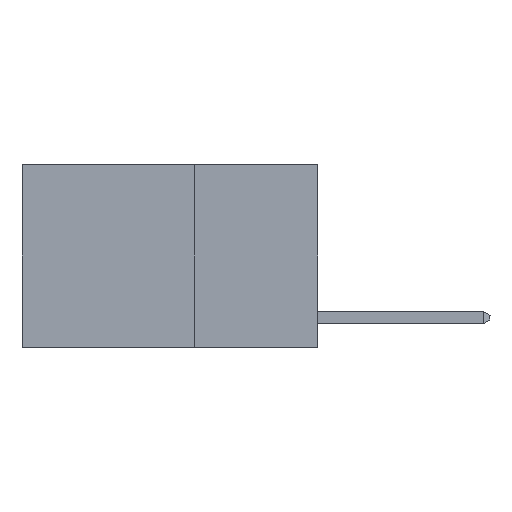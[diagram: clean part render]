
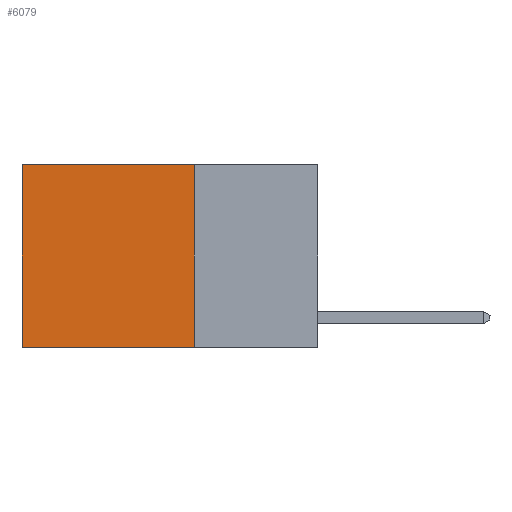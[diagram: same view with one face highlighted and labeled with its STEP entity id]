
A CAD part, left-side view. The second image highlights one B-rep face of the part: STEP entity #6079.
In plain terms, the highlighted planar face has unit normal (-1, 0, 0).
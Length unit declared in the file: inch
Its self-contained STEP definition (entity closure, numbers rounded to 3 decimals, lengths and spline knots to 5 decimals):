
#65 = LINE ( 'NONE', #15000, #6848 ) ;
#456 = VERTEX_POINT ( 'NONE', #9681 ) ;
#506 = EDGE_CURVE ( 'NONE', #2422, #10743, #3334, .T. ) ;
#2422 = VERTEX_POINT ( 'NONE', #9698 ) ;
#2647 = EDGE_CURVE ( 'NONE', #456, #5254, #65, .T. ) ;
#2948 = VECTOR ( 'NONE', #9373, 39.37008 ) ;
#2974 = ORIENTED_EDGE ( 'NONE', *, *, #14936, .F. ) ;
#2992 = DIRECTION ( 'NONE',  ( 0., 0., -1. ) ) ;
#3334 = LINE ( 'NONE', #9472, #2948 ) ;
#3987 = DIRECTION ( 'NONE',  ( 1., 0., 0. ) ) ;
#4174 = LINE ( 'NONE', #11429, #4573 ) ;
#4189 = ORIENTED_EDGE ( 'NONE', *, *, #7579, .T. ) ;
#4573 = VECTOR ( 'NONE', #2992, 39.37008 ) ;
#5254 = VERTEX_POINT ( 'NONE', #10690 ) ;
#6079 = ADVANCED_FACE ( 'NONE', ( #9887 ), #11171, .F. ) ;
#6286 = AXIS2_PLACEMENT_3D ( 'NONE', #8864, #3987, #12351 ) ;
#6848 = VECTOR ( 'NONE', #14938, 39.37008 ) ;
#7579 = EDGE_CURVE ( 'NONE', #5254, #10743, #13871, .T. ) ;
#7671 = VECTOR ( 'NONE', #13179, 39.37008 ) ;
#8773 = ORIENTED_EDGE ( 'NONE', *, *, #506, .F. ) ;
#8809 = ORIENTED_EDGE ( 'NONE', *, *, #2647, .T. ) ;
#8864 = CARTESIAN_POINT ( 'NONE',  ( 0.2625, 0.25, 0. ) ) ;
#9373 = DIRECTION ( 'NONE',  ( 0., 1., 0. ) ) ;
#9472 = CARTESIAN_POINT ( 'NONE',  ( 0.2625, 0.25, -0.37 ) ) ;
#9681 = CARTESIAN_POINT ( 'NONE',  ( 0.2625, 0.25, 0. ) ) ;
#9698 = CARTESIAN_POINT ( 'NONE',  ( 0.2625, 0.25, -0.37 ) ) ;
#9887 = FACE_OUTER_BOUND ( 'NONE', #11472, .T. ) ;
#10690 = CARTESIAN_POINT ( 'NONE',  ( 0.2625, 0.6, 0. ) ) ;
#10743 = VERTEX_POINT ( 'NONE', #13209 ) ;
#11171 = PLANE ( 'NONE',  #6286 ) ;
#11429 = CARTESIAN_POINT ( 'NONE',  ( 0.2625, 0.25, 0. ) ) ;
#11472 = EDGE_LOOP ( 'NONE', ( #4189, #8773, #2974, #8809 ) ) ;
#11949 = CARTESIAN_POINT ( 'NONE',  ( 0.2625, 0.6, 0. ) ) ;
#12351 = DIRECTION ( 'NONE',  ( 0., 0., -1. ) ) ;
#13179 = DIRECTION ( 'NONE',  ( 0., 0., -1. ) ) ;
#13209 = CARTESIAN_POINT ( 'NONE',  ( 0.2625, 0.6, -0.37 ) ) ;
#13871 = LINE ( 'NONE', #11949, #7671 ) ;
#14936 = EDGE_CURVE ( 'NONE', #456, #2422, #4174, .T. ) ;
#14938 = DIRECTION ( 'NONE',  ( 0., 1., 0. ) ) ;
#15000 = CARTESIAN_POINT ( 'NONE',  ( 0.2625, 0.25, 0. ) ) ;
